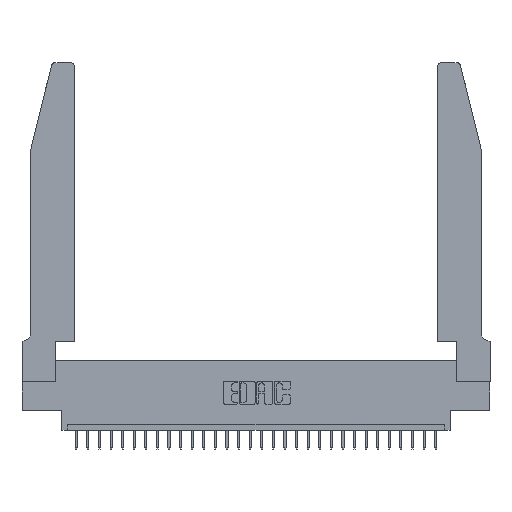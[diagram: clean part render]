
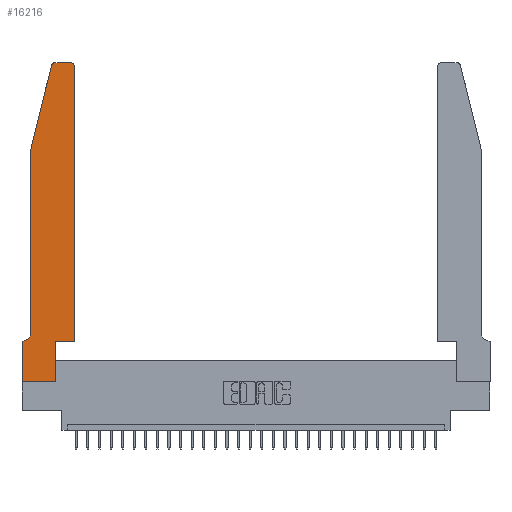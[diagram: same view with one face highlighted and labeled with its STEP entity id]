
A CAD part, top view. The second image highlights one B-rep face of the part: STEP entity #16216.
In plain terms, the highlighted planar face has unit normal (0, 0, 1).
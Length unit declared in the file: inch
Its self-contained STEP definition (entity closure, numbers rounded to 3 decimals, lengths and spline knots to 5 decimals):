
#321 = VERTEX_POINT ( 'NONE', #10119 ) ;
#559 = DIRECTION ( 'NONE',  ( 0., -1., 0. ) ) ;
#654 = VECTOR ( 'NONE', #19784, 39.37008 ) ;
#773 = CARTESIAN_POINT ( 'NONE',  ( 0.0755, 2., 0.37 ) ) ;
#2205 = CARTESIAN_POINT ( 'NONE',  ( 0.4205, 2.72, 0.37 ) ) ;
#2547 = CARTESIAN_POINT ( 'NONE',  ( 0.0755, 0.42, 0.37 ) ) ;
#2790 = ORIENTED_EDGE ( 'NONE', *, *, #6295, .T. ) ;
#2902 = VECTOR ( 'NONE', #17621, 39.37008 ) ;
#3336 = DIRECTION ( 'NONE',  ( 0., 0., 1. ) ) ;
#3754 = LINE ( 'NONE', #27614, #22127 ) ;
#3778 = EDGE_CURVE ( 'NONE', #20721, #17589, #21937, .T. ) ;
#3843 = CARTESIAN_POINT ( 'NONE',  ( 0., 0.35, 0.37 ) ) ;
#4027 = DIRECTION ( 'NONE',  ( -0.239, -0.971, 0. ) ) ;
#4049 = ORIENTED_EDGE ( 'NONE', *, *, #19463, .T. ) ;
#4282 = DIRECTION ( 'NONE',  ( 0., 0., 1. ) ) ;
#4975 = VECTOR ( 'NONE', #559, 39.37008 ) ;
#4980 = LINE ( 'NONE', #15991, #27666 ) ;
#5371 = VERTEX_POINT ( 'NONE', #2547 ) ;
#5489 = CARTESIAN_POINT ( 'NONE',  ( 0.0055, 0.42, 0.37 ) ) ;
#5509 = LINE ( 'NONE', #29198, #15742 ) ;
#5828 = VERTEX_POINT ( 'NONE', #30093 ) ;
#6022 = CARTESIAN_POINT ( 'NONE',  ( 0., 0., 0.37 ) ) ;
#6295 = EDGE_CURVE ( 'NONE', #5828, #28107, #13153, .T. ) ;
#6562 = CARTESIAN_POINT ( 'NONE',  ( 0.2865, 0.35, 0.37 ) ) ;
#7748 = EDGE_CURVE ( 'NONE', #5371, #5828, #12319, .T. ) ;
#8150 = CARTESIAN_POINT ( 'NONE',  ( 0.284, 2.72, 0.37 ) ) ;
#8241 = LINE ( 'NONE', #12267, #4975 ) ;
#8278 = EDGE_CURVE ( 'NONE', #16875, #5371, #8241, .T. ) ;
#8437 = ORIENTED_EDGE ( 'NONE', *, *, #20422, .T. ) ;
#8525 = VECTOR ( 'NONE', #22229, 39.37008 ) ;
#8734 = VECTOR ( 'NONE', #12303, 39.37008 ) ;
#8928 = ORIENTED_EDGE ( 'NONE', *, *, #18439, .T. ) ;
#8996 = EDGE_CURVE ( 'NONE', #17589, #16875, #4980, .T. ) ;
#9180 = DIRECTION ( 'NONE',  ( 0., 1., 0. ) ) ;
#9477 = ORIENTED_EDGE ( 'NONE', *, *, #7748, .T. ) ;
#10119 = CARTESIAN_POINT ( 'NONE',  ( 0.4505, 0.35, 0.37 ) ) ;
#10680 = CARTESIAN_POINT ( 'NONE',  ( 0.2605, 2.75, 0.37 ) ) ;
#11097 = ORIENTED_EDGE ( 'NONE', *, *, #3778, .T. ) ;
#11289 = LINE ( 'NONE', #26679, #8734 ) ;
#11383 = CARTESIAN_POINT ( 'NONE',  ( 0.4505, 0.35, 0.37 ) ) ;
#11422 = DIRECTION ( 'NONE',  ( 1., 0., 0. ) ) ;
#12027 = VERTEX_POINT ( 'NONE', #17232 ) ;
#12267 = CARTESIAN_POINT ( 'NONE',  ( 0.0755, 2., 0.37 ) ) ;
#12303 = DIRECTION ( 'NONE',  ( 0., 1., 0. ) ) ;
#12319 = CIRCLE ( 'NONE', #27882, 0.07 ) ;
#12341 = ORIENTED_EDGE ( 'NONE', *, *, #12586, .T. ) ;
#12586 = EDGE_CURVE ( 'NONE', #321, #12027, #3754, .T. ) ;
#13153 = LINE ( 'NONE', #24196, #654 ) ;
#13483 = CARTESIAN_POINT ( 'NONE',  ( 0.2865, 0., 0.37 ) ) ;
#13497 = EDGE_LOOP ( 'NONE', ( #22431, #11097, #27162, #26805, #9477, #2790, #4049, #18884, #26161, #8437, #12341, #8928 ) ) ;
#14714 = CARTESIAN_POINT ( 'NONE',  ( 0.4205, 2.75, 0.37 ) ) ;
#15319 = EDGE_CURVE ( 'NONE', #28145, #17772, #11289, .T. ) ;
#15371 = LINE ( 'NONE', #10680, #2902 ) ;
#15742 = VECTOR ( 'NONE', #29587, 39.37008 ) ;
#15991 = CARTESIAN_POINT ( 'NONE',  ( 0.0755, 2., 0.37 ) ) ;
#16216 = ADVANCED_FACE ( 'NONE', ( #27774 ), #23339, .T. ) ;
#16872 = VECTOR ( 'NONE', #20620, 39.37008 ) ;
#16875 = VERTEX_POINT ( 'NONE', #773 ) ;
#17232 = CARTESIAN_POINT ( 'NONE',  ( 0.4505, 2.72, 0.37 ) ) ;
#17589 = VERTEX_POINT ( 'NONE', #17921 ) ;
#17621 = DIRECTION ( 'NONE',  ( -1., 0., 0. ) ) ;
#17688 = VERTEX_POINT ( 'NONE', #27261 ) ;
#17772 = VERTEX_POINT ( 'NONE', #6562 ) ;
#17921 = CARTESIAN_POINT ( 'NONE',  ( 0.25487, 2.72718, 0.37 ) ) ;
#17977 = AXIS2_PLACEMENT_3D ( 'NONE', #2205, #4282, #25298 ) ;
#18439 = EDGE_CURVE ( 'NONE', #12027, #26378, #24367, .T. ) ;
#18884 = ORIENTED_EDGE ( 'NONE', *, *, #24144, .T. ) ;
#19463 = EDGE_CURVE ( 'NONE', #28107, #17688, #27240, .T. ) ;
#19784 = DIRECTION ( 'NONE',  ( -1., 0., 0. ) ) ;
#20422 = EDGE_CURVE ( 'NONE', #17772, #321, #23867, .T. ) ;
#20620 = DIRECTION ( 'NONE',  ( 1., 0., 0. ) ) ;
#20721 = VERTEX_POINT ( 'NONE', #21829 ) ;
#21070 = CARTESIAN_POINT ( 'NONE',  ( 0., 0.35, 0.37 ) ) ;
#21195 = EDGE_CURVE ( 'NONE', #26378, #20721, #15371, .T. ) ;
#21829 = CARTESIAN_POINT ( 'NONE',  ( 0.284, 2.75, 0.37 ) ) ;
#21890 = DIRECTION ( 'NONE',  ( 0., 0., -1. ) ) ;
#21937 = CIRCLE ( 'NONE', #24270, 0.03 ) ;
#22114 = DIRECTION ( 'NONE',  ( 1., 0., 0. ) ) ;
#22127 = VECTOR ( 'NONE', #9180, 39.37008 ) ;
#22229 = DIRECTION ( 'NONE',  ( 0., -1., 0. ) ) ;
#22431 = ORIENTED_EDGE ( 'NONE', *, *, #21195, .T. ) ;
#23339 = PLANE ( 'NONE',  #24225 ) ;
#23867 = LINE ( 'NONE', #11383, #16872 ) ;
#24144 = EDGE_CURVE ( 'NONE', #17688, #28145, #5509, .T. ) ;
#24196 = CARTESIAN_POINT ( 'NONE',  ( 0.0755, 0.35, 0.37 ) ) ;
#24225 = AXIS2_PLACEMENT_3D ( 'NONE', #21070, #25676, #11422 ) ;
#24270 = AXIS2_PLACEMENT_3D ( 'NONE', #8150, #3336, #22114 ) ;
#24367 = CIRCLE ( 'NONE', #17977, 0.03 ) ;
#24641 = DIRECTION ( 'NONE',  ( -1., 0., 0. ) ) ;
#25298 = DIRECTION ( 'NONE',  ( 1., 0., 0. ) ) ;
#25676 = DIRECTION ( 'NONE',  ( 0., 0., 1. ) ) ;
#26161 = ORIENTED_EDGE ( 'NONE', *, *, #15319, .T. ) ;
#26378 = VERTEX_POINT ( 'NONE', #14714 ) ;
#26679 = CARTESIAN_POINT ( 'NONE',  ( 0.2865, 0.35, 0.37 ) ) ;
#26805 = ORIENTED_EDGE ( 'NONE', *, *, #8278, .T. ) ;
#27162 = ORIENTED_EDGE ( 'NONE', *, *, #8996, .T. ) ;
#27240 = LINE ( 'NONE', #6022, #8525 ) ;
#27261 = CARTESIAN_POINT ( 'NONE',  ( 0., 0., 0.37 ) ) ;
#27614 = CARTESIAN_POINT ( 'NONE',  ( 0.4505, 0.35, 0.37 ) ) ;
#27666 = VECTOR ( 'NONE', #4027, 39.37008 ) ;
#27774 = FACE_OUTER_BOUND ( 'NONE', #13497, .T. ) ;
#27882 = AXIS2_PLACEMENT_3D ( 'NONE', #5489, #21890, #24641 ) ;
#28107 = VERTEX_POINT ( 'NONE', #3843 ) ;
#28145 = VERTEX_POINT ( 'NONE', #13483 ) ;
#29198 = CARTESIAN_POINT ( 'NONE',  ( 0., 0., 0.37 ) ) ;
#29587 = DIRECTION ( 'NONE',  ( 1., 0., 0. ) ) ;
#30093 = CARTESIAN_POINT ( 'NONE',  ( 0.0055, 0.35, 0.37 ) ) ;
